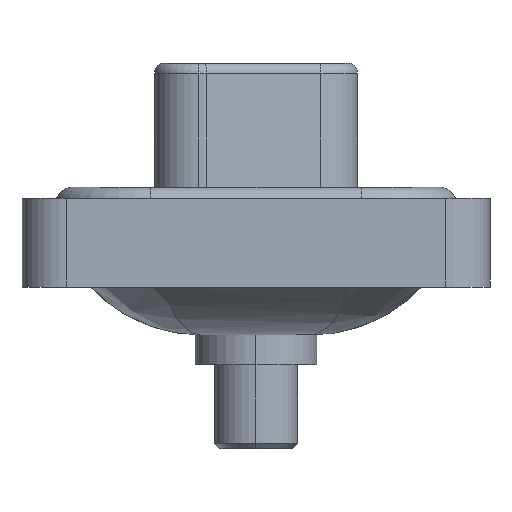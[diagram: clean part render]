
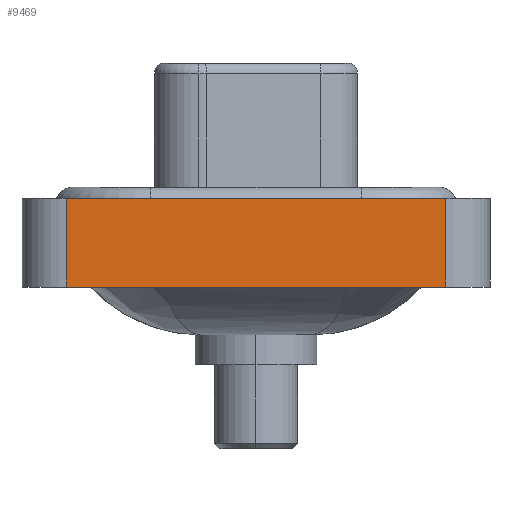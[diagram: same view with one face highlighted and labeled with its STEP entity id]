
A CAD part, left-side view. The second image highlights one B-rep face of the part: STEP entity #9469.
In plain terms, the highlighted planar face has unit normal (-1, 0, 0).
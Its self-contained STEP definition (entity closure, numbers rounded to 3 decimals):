
#920 = FACE_OUTER_BOUND ( 'NONE', #13533, .T. ) ;
#1260 = EDGE_CURVE ( 'NONE', #4745, #4866, #8161, .T. ) ;
#1791 = ORIENTED_EDGE ( 'NONE', *, *, #13007, .T. ) ;
#2301 = LINE ( 'NONE', #12878, #11604 ) ;
#3230 = ORIENTED_EDGE ( 'NONE', *, *, #1260, .T. ) ;
#3253 = LINE ( 'NONE', #11585, #5415 ) ;
#3479 = ORIENTED_EDGE ( 'NONE', *, *, #12786, .F. ) ;
#3924 = EDGE_CURVE ( 'NONE', #7856, #5860, #4330, .T. ) ;
#4330 = LINE ( 'NONE', #13908, #7759 ) ;
#4574 = DIRECTION ( 'NONE',  ( 0., -1., 0. ) ) ;
#4745 = VERTEX_POINT ( 'NONE', #11399 ) ;
#4866 = VERTEX_POINT ( 'NONE', #11856 ) ;
#5415 = VECTOR ( 'NONE', #4574, 1000. ) ;
#5860 = VERTEX_POINT ( 'NONE', #12488 ) ;
#6833 = PLANE ( 'NONE',  #9820 ) ;
#6955 = CARTESIAN_POINT ( 'NONE',  ( -7.25, 8.55, -3.6 ) ) ;
#6981 = DIRECTION ( 'NONE',  ( -1., 0., 0. ) ) ;
#7759 = VECTOR ( 'NONE', #13745, 1000. ) ;
#7856 = VERTEX_POINT ( 'NONE', #6955 ) ;
#8161 = LINE ( 'NONE', #12861, #8952 ) ;
#8190 = CARTESIAN_POINT ( 'NONE',  ( -7.25, -8.55, -3.6 ) ) ;
#8952 = VECTOR ( 'NONE', #15271, 1000. ) ;
#9469 = ADVANCED_FACE ( 'NONE', ( #920 ), #6833, .T. ) ;
#9820 = AXIS2_PLACEMENT_3D ( 'NONE', #8190, #6981, #10425 ) ;
#10425 = DIRECTION ( 'NONE',  ( 0., 0., 1. ) ) ;
#11399 = CARTESIAN_POINT ( 'NONE',  ( -7.25, -8.55, -3.6 ) ) ;
#11585 = CARTESIAN_POINT ( 'NONE',  ( -7.25, -8.55, -3.6 ) ) ;
#11604 = VECTOR ( 'NONE', #12735, 1000. ) ;
#11856 = CARTESIAN_POINT ( 'NONE',  ( -7.25, -8.55, 0.4 ) ) ;
#12488 = CARTESIAN_POINT ( 'NONE',  ( -7.25, 8.55, 0.4 ) ) ;
#12735 = DIRECTION ( 'NONE',  ( 0., -1., 0. ) ) ;
#12786 = EDGE_CURVE ( 'NONE', #5860, #4866, #2301, .T. ) ;
#12861 = CARTESIAN_POINT ( 'NONE',  ( -7.25, -8.55, -3.6 ) ) ;
#12878 = CARTESIAN_POINT ( 'NONE',  ( -7.25, -8.55, 0.4 ) ) ;
#13007 = EDGE_CURVE ( 'NONE', #7856, #4745, #3253, .T. ) ;
#13533 = EDGE_LOOP ( 'NONE', ( #3230, #3479, #13670, #1791 ) ) ;
#13670 = ORIENTED_EDGE ( 'NONE', *, *, #3924, .F. ) ;
#13745 = DIRECTION ( 'NONE',  ( 0., 0., 1. ) ) ;
#13908 = CARTESIAN_POINT ( 'NONE',  ( -7.25, 8.55, -3.6 ) ) ;
#15271 = DIRECTION ( 'NONE',  ( 0., 0., 1. ) ) ;
